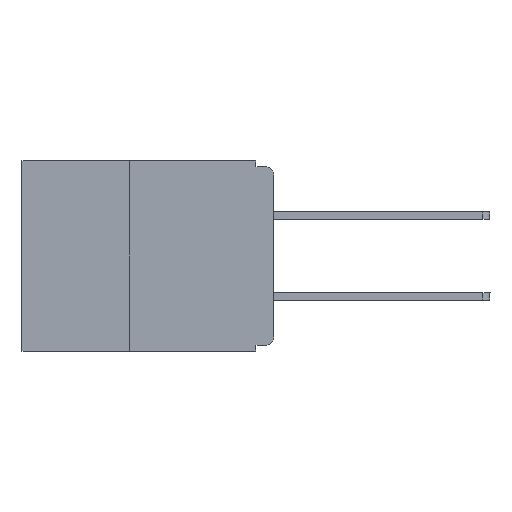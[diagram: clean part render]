
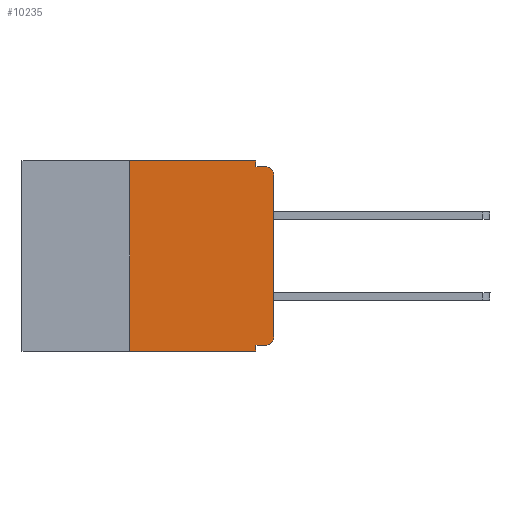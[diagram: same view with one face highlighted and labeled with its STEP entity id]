
A CAD part, left-side view. The second image highlights one B-rep face of the part: STEP entity #10235.
In plain terms, the highlighted planar face has unit normal (-1, 0, 0).
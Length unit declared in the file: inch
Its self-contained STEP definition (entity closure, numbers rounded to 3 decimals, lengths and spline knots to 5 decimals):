
#737 = ORIENTED_EDGE ( 'NONE', *, *, #9323, .T. ) ;
#842 = VERTEX_POINT ( 'NONE', #9372 ) ;
#853 = LINE ( 'NONE', #6767, #7573 ) ;
#865 = AXIS2_PLACEMENT_3D ( 'NONE', #5841, #10593, #9683 ) ;
#978 = CARTESIAN_POINT ( 'NONE',  ( 0., 0.437, -0.33 ) ) ;
#1062 = VERTEX_POINT ( 'NONE', #9031 ) ;
#1269 = EDGE_CURVE ( 'NONE', #4936, #842, #853, .T. ) ;
#1276 = VERTEX_POINT ( 'NONE', #4951 ) ;
#1357 = DIRECTION ( 'NONE',  ( 0., 0., -1. ) ) ;
#1899 = EDGE_CURVE ( 'NONE', #11282, #9777, #5475, .T. ) ;
#2001 = DIRECTION ( 'NONE',  ( 0., 0., -1. ) ) ;
#2181 = PLANE ( 'NONE',  #865 ) ;
#2611 = EDGE_CURVE ( 'NONE', #842, #4629, #10316, .T. ) ;
#2672 = VECTOR ( 'NONE', #2001, 39.37008 ) ;
#2674 = ORIENTED_EDGE ( 'NONE', *, *, #6405, .F. ) ;
#2745 = DIRECTION ( 'NONE',  ( 0., -1., 0. ) ) ;
#3056 = ORIENTED_EDGE ( 'NONE', *, *, #2611, .F. ) ;
#3136 = CARTESIAN_POINT ( 'NONE',  ( 0., 0.031, -0.33 ) ) ;
#3252 = AXIS2_PLACEMENT_3D ( 'NONE', #4173, #6985, #1357 ) ;
#3412 = ORIENTED_EDGE ( 'NONE', *, *, #7731, .F. ) ;
#3578 = ORIENTED_EDGE ( 'NONE', *, *, #1269, .F. ) ;
#3652 = FACE_OUTER_BOUND ( 'NONE', #6093, .T. ) ;
#3694 = AXIS2_PLACEMENT_3D ( 'NONE', #4147, #11701, #11742 ) ;
#4147 = CARTESIAN_POINT ( 'NONE',  ( 0., 0.015, -0.305 ) ) ;
#4154 = VECTOR ( 'NONE', #6122, 39.37008 ) ;
#4173 = CARTESIAN_POINT ( 'NONE',  ( 0., 0.015, -0.025 ) ) ;
#4373 = CARTESIAN_POINT ( 'NONE',  ( 0., 0.25, -0.33 ) ) ;
#4629 = VERTEX_POINT ( 'NONE', #10756 ) ;
#4936 = VERTEX_POINT ( 'NONE', #11256 ) ;
#4951 = CARTESIAN_POINT ( 'NONE',  ( 0., 0., -0.025 ) ) ;
#5196 = CARTESIAN_POINT ( 'NONE',  ( 0., 0., -0.01 ) ) ;
#5475 = LINE ( 'NONE', #10371, #2672 ) ;
#5618 = EDGE_CURVE ( 'NONE', #10800, #9777, #6437, .T. ) ;
#5841 = CARTESIAN_POINT ( 'NONE',  ( 0., 0.437, 0. ) ) ;
#6073 = LINE ( 'NONE', #11007, #4154 ) ;
#6093 = EDGE_LOOP ( 'NONE', ( #737, #7456, #3056, #3578, #3412, #2674, #9537, #7881, #8434, #9576 ) ) ;
#6122 = DIRECTION ( 'NONE',  ( 0., 1., 0. ) ) ;
#6231 = VECTOR ( 'NONE', #2745, 39.37008 ) ;
#6364 = DIRECTION ( 'NONE',  ( 0., -1., 0. ) ) ;
#6405 = EDGE_CURVE ( 'NONE', #10800, #1062, #8164, .T. ) ;
#6437 = LINE ( 'NONE', #978, #9824 ) ;
#6573 = CARTESIAN_POINT ( 'NONE',  ( 0., 0.437, 0. ) ) ;
#6767 = CARTESIAN_POINT ( 'NONE',  ( 0., 0.031, 0. ) ) ;
#6920 = EDGE_CURVE ( 'NONE', #8439, #7494, #8891, .T. ) ;
#6985 = DIRECTION ( 'NONE',  ( -1., 0., 0. ) ) ;
#7199 = CIRCLE ( 'NONE', #3252, 0.015 ) ;
#7248 = CARTESIAN_POINT ( 'NONE',  ( 0., 0.031, -0.32 ) ) ;
#7296 = DIRECTION ( 'NONE',  ( 0., 0., 1. ) ) ;
#7442 = VECTOR ( 'NONE', #11922, 39.37008 ) ;
#7456 = ORIENTED_EDGE ( 'NONE', *, *, #11866, .T. ) ;
#7494 = VERTEX_POINT ( 'NONE', #8954 ) ;
#7573 = VECTOR ( 'NONE', #10550, 39.37008 ) ;
#7731 = EDGE_CURVE ( 'NONE', #1062, #4936, #11832, .T. ) ;
#7881 = ORIENTED_EDGE ( 'NONE', *, *, #1899, .F. ) ;
#8139 = EDGE_CURVE ( 'NONE', #8439, #11282, #6073, .T. ) ;
#8164 = LINE ( 'NONE', #4373, #7442 ) ;
#8434 = ORIENTED_EDGE ( 'NONE', *, *, #8139, .F. ) ;
#8439 = VERTEX_POINT ( 'NONE', #8464 ) ;
#8464 = CARTESIAN_POINT ( 'NONE',  ( 0., 0.015, -0.32 ) ) ;
#8683 = VECTOR ( 'NONE', #7296, 39.37008 ) ;
#8891 = CIRCLE ( 'NONE', #3694, 0.015 ) ;
#8954 = CARTESIAN_POINT ( 'NONE',  ( 0., 0., -0.305 ) ) ;
#9031 = CARTESIAN_POINT ( 'NONE',  ( 0., 0.25, 0. ) ) ;
#9298 = CARTESIAN_POINT ( 'NONE',  ( 0., 0., 0. ) ) ;
#9323 = EDGE_CURVE ( 'NONE', #7494, #1276, #11952, .T. ) ;
#9372 = CARTESIAN_POINT ( 'NONE',  ( 0., 0.031, -0.01 ) ) ;
#9419 = DIRECTION ( 'NONE',  ( 0., -1., 0. ) ) ;
#9519 = CARTESIAN_POINT ( 'NONE',  ( 0., 0.25, -0.33 ) ) ;
#9537 = ORIENTED_EDGE ( 'NONE', *, *, #5618, .T. ) ;
#9576 = ORIENTED_EDGE ( 'NONE', *, *, #6920, .T. ) ;
#9683 = DIRECTION ( 'NONE',  ( 0., 0., -1. ) ) ;
#9777 = VERTEX_POINT ( 'NONE', #3136 ) ;
#9824 = VECTOR ( 'NONE', #9419, 39.37008 ) ;
#10235 = ADVANCED_FACE ( 'NONE', ( #3652 ), #2181, .F. ) ;
#10316 = LINE ( 'NONE', #5196, #10615 ) ;
#10371 = CARTESIAN_POINT ( 'NONE',  ( 0., 0.031, -0.33 ) ) ;
#10550 = DIRECTION ( 'NONE',  ( 0., 0., -1. ) ) ;
#10593 = DIRECTION ( 'NONE',  ( 1., 0., 0. ) ) ;
#10615 = VECTOR ( 'NONE', #6364, 39.37008 ) ;
#10756 = CARTESIAN_POINT ( 'NONE',  ( 0., 0.015, -0.01 ) ) ;
#10800 = VERTEX_POINT ( 'NONE', #9519 ) ;
#11007 = CARTESIAN_POINT ( 'NONE',  ( 0., 0., -0.32 ) ) ;
#11256 = CARTESIAN_POINT ( 'NONE',  ( 0., 0.031, 0. ) ) ;
#11282 = VERTEX_POINT ( 'NONE', #7248 ) ;
#11701 = DIRECTION ( 'NONE',  ( -1., 0., 0. ) ) ;
#11742 = DIRECTION ( 'NONE',  ( 0., 0., -1. ) ) ;
#11832 = LINE ( 'NONE', #6573, #6231 ) ;
#11866 = EDGE_CURVE ( 'NONE', #1276, #4629, #7199, .T. ) ;
#11922 = DIRECTION ( 'NONE',  ( 0., 0., 1. ) ) ;
#11952 = LINE ( 'NONE', #9298, #8683 ) ;
